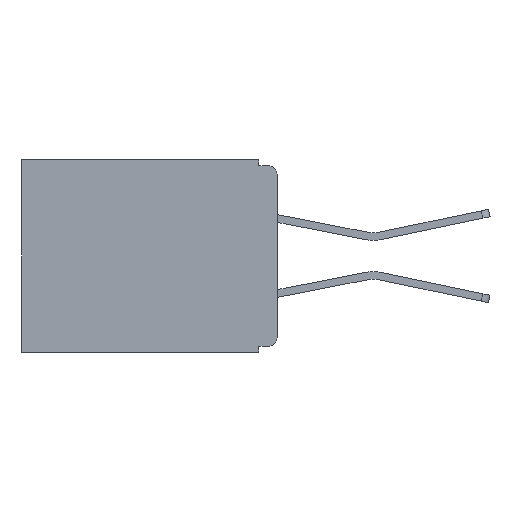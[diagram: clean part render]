
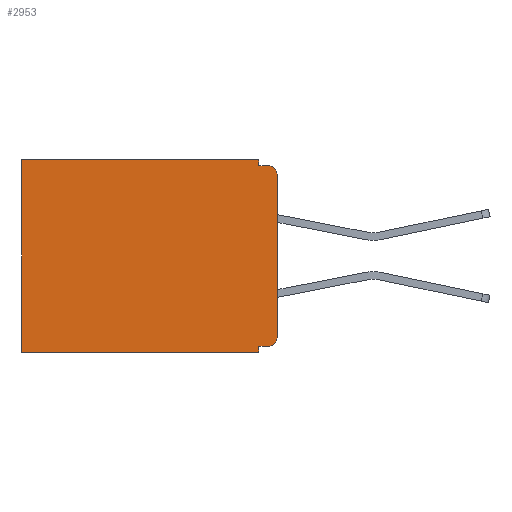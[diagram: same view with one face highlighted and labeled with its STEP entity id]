
A CAD part, left-side view. The second image highlights one B-rep face of the part: STEP entity #2953.
In plain terms, the highlighted planar face has unit normal (-1, 0, 0).
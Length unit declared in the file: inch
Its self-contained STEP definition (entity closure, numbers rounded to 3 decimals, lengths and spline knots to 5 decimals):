
#97 = AXIS2_PLACEMENT_3D ( 'NONE', #16086, #5900, #18067 ) ;
#98 = VECTOR ( 'NONE', #20099, 39.37008 ) ;
#162 = CARTESIAN_POINT ( 'NONE',  ( 0.3, 0.031, 0. ) ) ;
#171 = VERTEX_POINT ( 'NONE', #14474 ) ;
#178 = CARTESIAN_POINT ( 'NONE',  ( 0.3, 0.031, -0.33 ) ) ;
#773 = LINE ( 'NONE', #13148, #5068 ) ;
#942 = VERTEX_POINT ( 'NONE', #18901 ) ;
#1439 = EDGE_CURVE ( 'NONE', #5255, #6882, #7939, .T. ) ;
#1504 = CARTESIAN_POINT ( 'NONE',  ( 0.3, 0., -0.305 ) ) ;
#2050 = DIRECTION ( 'NONE',  ( 0., 0., -1. ) ) ;
#2208 = DIRECTION ( 'NONE',  ( 0., 0., -1. ) ) ;
#2367 = VECTOR ( 'NONE', #22304, 39.37008 ) ;
#2625 = VERTEX_POINT ( 'NONE', #11983 ) ;
#2804 = VERTEX_POINT ( 'NONE', #162 ) ;
#2953 = ADVANCED_FACE ( 'NONE', ( #15535 ), #19390, .F. ) ;
#3028 = CARTESIAN_POINT ( 'NONE',  ( 0.3, 0.031, -0.01 ) ) ;
#3271 = DIRECTION ( 'NONE',  ( 0., 0., -1. ) ) ;
#3431 = CARTESIAN_POINT ( 'NONE',  ( 0.3, 0., -0.025 ) ) ;
#3754 = CARTESIAN_POINT ( 'NONE',  ( 0.3, 0., -0.33 ) ) ;
#3847 = CARTESIAN_POINT ( 'NONE',  ( 0.3, 0.437, -0.33 ) ) ;
#3897 = EDGE_CURVE ( 'NONE', #11955, #2625, #20991, .T. ) ;
#4243 = LINE ( 'NONE', #3754, #8450 ) ;
#4982 = LINE ( 'NONE', #7982, #98 ) ;
#5068 = VECTOR ( 'NONE', #13009, 39.37008 ) ;
#5255 = VERTEX_POINT ( 'NONE', #14337 ) ;
#5460 = DIRECTION ( 'NONE',  ( -1., 0., 0. ) ) ;
#5900 = DIRECTION ( 'NONE',  ( -1., 0., 0. ) ) ;
#6132 = CARTESIAN_POINT ( 'NONE',  ( 0.3, 0.015, -0.305 ) ) ;
#6353 = VECTOR ( 'NONE', #6381, 39.37008 ) ;
#6381 = DIRECTION ( 'NONE',  ( 0., 1., 0. ) ) ;
#6705 = CARTESIAN_POINT ( 'NONE',  ( 0.3, 0.031, 0. ) ) ;
#6882 = VERTEX_POINT ( 'NONE', #1504 ) ;
#7492 = EDGE_CURVE ( 'NONE', #5255, #942, #773, .T. ) ;
#7939 = CIRCLE ( 'NONE', #20602, 0.015 ) ;
#7982 = CARTESIAN_POINT ( 'NONE',  ( 0.3, 0., -0.01 ) ) ;
#8179 = CARTESIAN_POINT ( 'NONE',  ( 0.3, 0., 0. ) ) ;
#8305 = EDGE_CURVE ( 'NONE', #20155, #15757, #11941, .T. ) ;
#8450 = VECTOR ( 'NONE', #17806, 39.37008 ) ;
#8583 = CARTESIAN_POINT ( 'NONE',  ( 0.3, 0.437, -0.33 ) ) ;
#8845 = EDGE_CURVE ( 'NONE', #2804, #20155, #15746, .T. ) ;
#8919 = LINE ( 'NONE', #178, #13113 ) ;
#11278 = CARTESIAN_POINT ( 'NONE',  ( 0.3, 0., -0.33 ) ) ;
#11941 = LINE ( 'NONE', #8583, #2367 ) ;
#11955 = VERTEX_POINT ( 'NONE', #3431 ) ;
#11983 = CARTESIAN_POINT ( 'NONE',  ( 0.3, 0.015, -0.01 ) ) ;
#12488 = ORIENTED_EDGE ( 'NONE', *, *, #19467, .F. ) ;
#12512 = ORIENTED_EDGE ( 'NONE', *, *, #3897, .T. ) ;
#12886 = ORIENTED_EDGE ( 'NONE', *, *, #13807, .F. ) ;
#12904 = ORIENTED_EDGE ( 'NONE', *, *, #14754, .F. ) ;
#13009 = DIRECTION ( 'NONE',  ( 0., 1., 0. ) ) ;
#13113 = VECTOR ( 'NONE', #2050, 39.37008 ) ;
#13148 = CARTESIAN_POINT ( 'NONE',  ( 0.3, 0., -0.32 ) ) ;
#13167 = ORIENTED_EDGE ( 'NONE', *, *, #8845, .T. ) ;
#13194 = ORIENTED_EDGE ( 'NONE', *, *, #8305, .T. ) ;
#13366 = ORIENTED_EDGE ( 'NONE', *, *, #22601, .F. ) ;
#13392 = ORIENTED_EDGE ( 'NONE', *, *, #13627, .F. ) ;
#13415 = ORIENTED_EDGE ( 'NONE', *, *, #7492, .F. ) ;
#13627 = EDGE_CURVE ( 'NONE', #942, #171, #8919, .T. ) ;
#13628 = ORIENTED_EDGE ( 'NONE', *, *, #1439, .T. ) ;
#13807 = EDGE_CURVE ( 'NONE', #17849, #2625, #4982, .T. ) ;
#14220 = VECTOR ( 'NONE', #17207, 39.37008 ) ;
#14337 = CARTESIAN_POINT ( 'NONE',  ( 0.3, 0.015, -0.32 ) ) ;
#14474 = CARTESIAN_POINT ( 'NONE',  ( 0.3, 0.031, -0.33 ) ) ;
#14584 = VECTOR ( 'NONE', #2208, 39.37008 ) ;
#14754 = EDGE_CURVE ( 'NONE', #2804, #17849, #19247, .T. ) ;
#15535 = FACE_OUTER_BOUND ( 'NONE', #18329, .T. ) ;
#15746 = LINE ( 'NONE', #8179, #6353 ) ;
#15757 = VERTEX_POINT ( 'NONE', #3847 ) ;
#16086 = CARTESIAN_POINT ( 'NONE',  ( 0.3, 0.015, -0.025 ) ) ;
#17207 = DIRECTION ( 'NONE',  ( 0., 0., -1. ) ) ;
#17806 = DIRECTION ( 'NONE',  ( 0., 1., 0. ) ) ;
#17849 = VERTEX_POINT ( 'NONE', #3028 ) ;
#18067 = DIRECTION ( 'NONE',  ( 0., 0., -1. ) ) ;
#18329 = EDGE_LOOP ( 'NONE', ( #12488, #12512, #12886, #12904, #13167, #13194, #13366, #13392, #13415, #13628 ) ) ;
#18512 = AXIS2_PLACEMENT_3D ( 'NONE', #19763, #19693, #19264 ) ;
#18901 = CARTESIAN_POINT ( 'NONE',  ( 0.3, 0.031, -0.32 ) ) ;
#19247 = LINE ( 'NONE', #6705, #14220 ) ;
#19264 = DIRECTION ( 'NONE',  ( 0., 0., -1. ) ) ;
#19390 = PLANE ( 'NONE',  #18512 ) ;
#19467 = EDGE_CURVE ( 'NONE', #11955, #6882, #20142, .T. ) ;
#19693 = DIRECTION ( 'NONE',  ( 1., 0., 0. ) ) ;
#19763 = CARTESIAN_POINT ( 'NONE',  ( 0.3, 0., -0.33 ) ) ;
#20099 = DIRECTION ( 'NONE',  ( 0., -1., 0. ) ) ;
#20142 = LINE ( 'NONE', #11278, #14584 ) ;
#20155 = VERTEX_POINT ( 'NONE', #21747 ) ;
#20602 = AXIS2_PLACEMENT_3D ( 'NONE', #6132, #5460, #3271 ) ;
#20991 = CIRCLE ( 'NONE', #97, 0.015 ) ;
#21747 = CARTESIAN_POINT ( 'NONE',  ( 0.3, 0.437, 0. ) ) ;
#22304 = DIRECTION ( 'NONE',  ( 0., 0., -1. ) ) ;
#22601 = EDGE_CURVE ( 'NONE', #171, #15757, #4243, .T. ) ;
